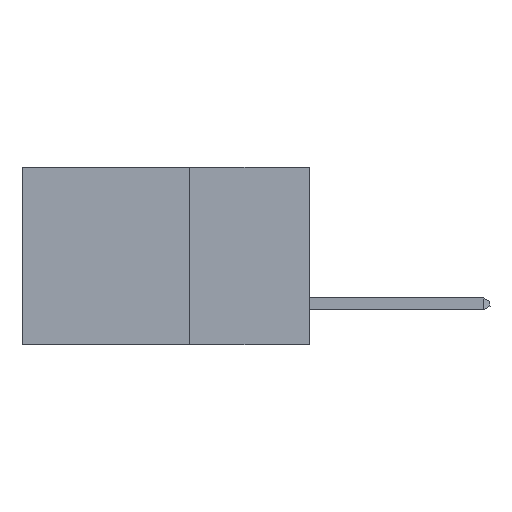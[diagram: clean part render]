
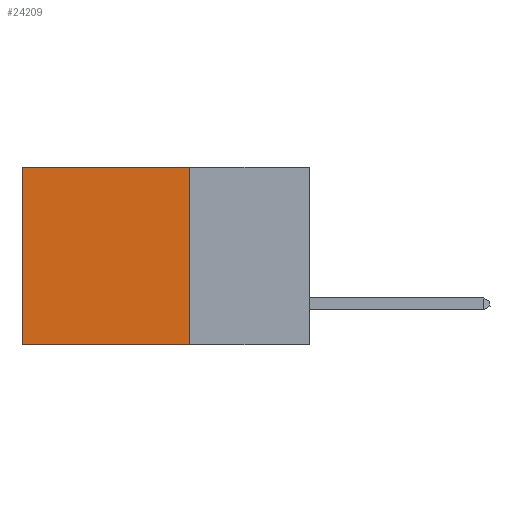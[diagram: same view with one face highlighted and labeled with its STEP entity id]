
A CAD part, left-side view. The second image highlights one B-rep face of the part: STEP entity #24209.
In plain terms, the highlighted planar face has unit normal (-1, 0, 0).
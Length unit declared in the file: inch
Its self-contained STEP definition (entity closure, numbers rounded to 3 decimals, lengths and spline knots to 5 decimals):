
#1136 = VERTEX_POINT ( 'NONE', #1371 ) ;
#1300 = DIRECTION ( 'NONE',  ( 0., 1., 0. ) ) ;
#1371 = CARTESIAN_POINT ( 'NONE',  ( 0.2875, 0.6, -0.37 ) ) ;
#1460 = VECTOR ( 'NONE', #25910, 39.37008 ) ;
#1965 = VERTEX_POINT ( 'NONE', #23034 ) ;
#2474 = ORIENTED_EDGE ( 'NONE', *, *, #34509, .T. ) ;
#2820 = VERTEX_POINT ( 'NONE', #27405 ) ;
#4531 = PLANE ( 'NONE',  #36952 ) ;
#5715 = EDGE_LOOP ( 'NONE', ( #2474, #12417, #12273, #31244 ) ) ;
#5866 = CARTESIAN_POINT ( 'NONE',  ( 0.2875, 0.25, -0.37 ) ) ;
#7486 = DIRECTION ( 'NONE',  ( 1., 0., 0. ) ) ;
#8654 = VECTOR ( 'NONE', #1300, 39.37008 ) ;
#12017 = VECTOR ( 'NONE', #31256, 39.37008 ) ;
#12273 = ORIENTED_EDGE ( 'NONE', *, *, #30221, .F. ) ;
#12417 = ORIENTED_EDGE ( 'NONE', *, *, #15079, .F. ) ;
#14575 = LINE ( 'NONE', #18822, #8654 ) ;
#15079 = EDGE_CURVE ( 'NONE', #35767, #1136, #14575, .T. ) ;
#16688 = DIRECTION ( 'NONE',  ( 0., 0., -1. ) ) ;
#16856 = LINE ( 'NONE', #25310, #26394 ) ;
#17035 = LINE ( 'NONE', #23008, #1460 ) ;
#18822 = CARTESIAN_POINT ( 'NONE',  ( 0.2875, 0.25, -0.37 ) ) ;
#18915 = FACE_OUTER_BOUND ( 'NONE', #5715, .T. ) ;
#22620 = CARTESIAN_POINT ( 'NONE',  ( 0.2875, 0.6, 0. ) ) ;
#23008 = CARTESIAN_POINT ( 'NONE',  ( 0.2875, 0.25, 0. ) ) ;
#23034 = CARTESIAN_POINT ( 'NONE',  ( 0.2875, 0.6, 0. ) ) ;
#24209 = ADVANCED_FACE ( 'NONE', ( #18915 ), #4531, .F. ) ;
#24858 = CARTESIAN_POINT ( 'NONE',  ( 0.2875, 0.25, 0. ) ) ;
#25310 = CARTESIAN_POINT ( 'NONE',  ( 0.2875, 0.25, 0. ) ) ;
#25784 = EDGE_CURVE ( 'NONE', #2820, #1965, #17035, .T. ) ;
#25910 = DIRECTION ( 'NONE',  ( 0., 1., 0. ) ) ;
#26394 = VECTOR ( 'NONE', #16688, 39.37008 ) ;
#27405 = CARTESIAN_POINT ( 'NONE',  ( 0.2875, 0.25, 0. ) ) ;
#27803 = DIRECTION ( 'NONE',  ( 0., 0., -1. ) ) ;
#30221 = EDGE_CURVE ( 'NONE', #2820, #35767, #16856, .T. ) ;
#31244 = ORIENTED_EDGE ( 'NONE', *, *, #25784, .T. ) ;
#31256 = DIRECTION ( 'NONE',  ( 0., 0., -1. ) ) ;
#34296 = LINE ( 'NONE', #22620, #12017 ) ;
#34509 = EDGE_CURVE ( 'NONE', #1965, #1136, #34296, .T. ) ;
#35767 = VERTEX_POINT ( 'NONE', #5866 ) ;
#36952 = AXIS2_PLACEMENT_3D ( 'NONE', #24858, #7486, #27803 ) ;
